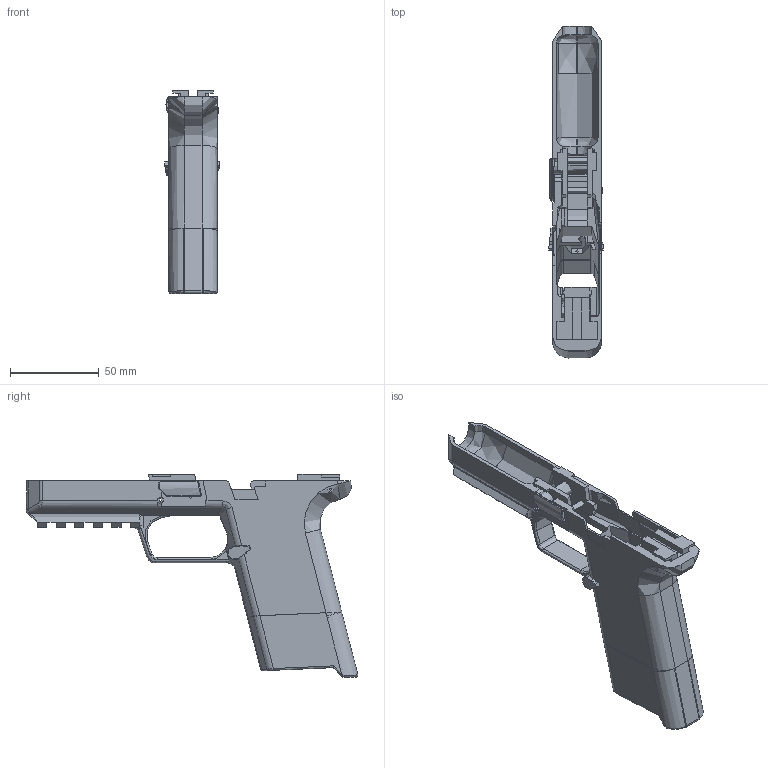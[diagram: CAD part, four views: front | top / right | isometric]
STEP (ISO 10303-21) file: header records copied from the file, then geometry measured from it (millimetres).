
FILE_DESCRIPTION(/* description */ (''),/* implementation_level */ '2;1');
FILE_NAME(/* name */ 'M&P 9 Assembly + Picatinny - Full Size Slide.step',/* time_stamp */ '2021-11-02T07:26:54-04:00',/* author */ (''),/* organization */ (''),/* preprocessor_version */ 'ST-DEVELOPER v18.1',/* originating_system */ 'Autodesk Translation Framework v10.10.0.1391',/* authorisation */ '');
FILE_SCHEMA (('AUTOMOTIVE_DESIGN { 1 0 10303 214 3 1 1 }'));
Length unit declared in the file: millimetre
Products named in the file (14): M&P 9 Standard Length Slide - Picatinny; M&P 9 Reference v94; Rear Fire Control Group Pin; Front Locking Block Group Pin; Trigger Pin; Locking Block; Disassembly Lug; Rear Fire Control Group; Frame; Trigger Guard and Magwell; Fitment Section; Nose; Magazine Release Button; Full-Size Magwell Body
Assembly tree (13 placements, depth 5):
  M&P 9 Standard Length Slide - Picatinny
    M&P 9 Reference v94
      Rear Fire Control Group Pin
      Front Locking Block Group Pin
      Trigger Pin
      Locking Block
      Disassembly Lug
      Rear Fire Control Group
      Frame
        Trigger Guard and Magwell
        Fitment Section
          Nose
        Magazine Release Button
        Full-Size Magwell Body
Bounding box: 30.85 x 187.13 x 114.63 mm (x, y, z)
Volume: 107801.6 mm3; surface area: 58819.5 mm2
Topology: 11 solids, 11 shells, 642 faces, 1754 edges, 1120 vertices
Faces by surface type: plane 356, cylinder 187, bspline 79, torus 15, sphere 4, cone 1
Full cylindrical faces by diameter (mm): 1.35 x2, 2 x3, 3.15 x2, 3.18 x3, 3.2 x2, 3.361 x2, 3.5 x1, 3.55 x4, 4.7 x1, 6.3 x1, 7.7 x1, 8.8 x1, 9 x2
Entity records: 23291 total; most frequent: CARTESIAN_POINT 6716, ORIENTED_EDGE 3500, DIRECTION 3263, EDGE_CURVE 1750, LINE 1131, VECTOR 1131, VERTEX_POINT 1120, AXIS2_PLACEMENT_3D 1066
